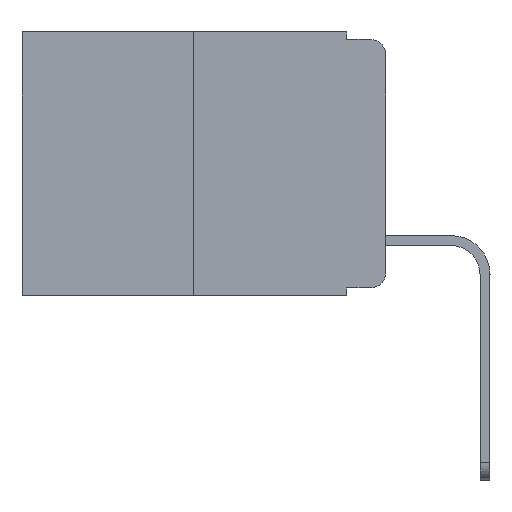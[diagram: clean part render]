
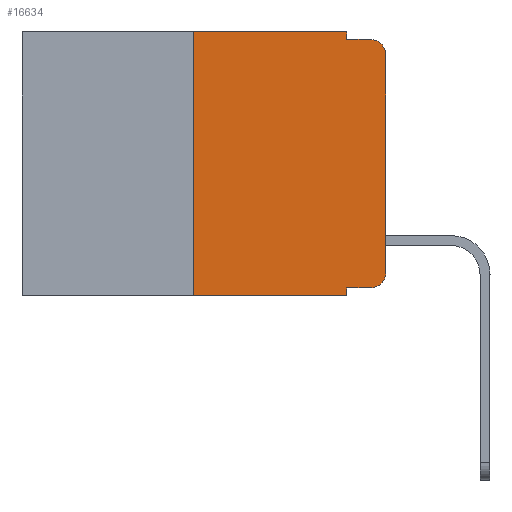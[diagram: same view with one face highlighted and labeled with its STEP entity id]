
A CAD part, left-side view. The second image highlights one B-rep face of the part: STEP entity #16634.
In plain terms, the highlighted planar face has unit normal (-1, 0, 0).
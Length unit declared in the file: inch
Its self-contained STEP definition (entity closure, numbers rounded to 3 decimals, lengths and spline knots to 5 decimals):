
#29 = VERTEX_POINT ( 'NONE', #22123 ) ;
#219 = LINE ( 'NONE', #21294, #9144 ) ;
#659 = ORIENTED_EDGE ( 'NONE', *, *, #23972, .F. ) ;
#1076 = CARTESIAN_POINT ( 'NONE',  ( 0., 0., 0. ) ) ;
#1132 = EDGE_CURVE ( 'NONE', #6059, #8301, #13253, .T. ) ;
#1584 = FACE_OUTER_BOUND ( 'NONE', #11433, .T. ) ;
#1598 = DIRECTION ( 'NONE',  ( -1., 0., 0. ) ) ;
#1832 = CARTESIAN_POINT ( 'NONE',  ( 0., 0.051, -0.01 ) ) ;
#2442 = VERTEX_POINT ( 'NONE', #19924 ) ;
#2556 = ORIENTED_EDGE ( 'NONE', *, *, #23384, .F. ) ;
#2822 = EDGE_CURVE ( 'NONE', #29, #23884, #219, .T. ) ;
#2874 = DIRECTION ( 'NONE',  ( 0., 0., -1. ) ) ;
#3214 = LINE ( 'NONE', #7345, #19552 ) ;
#3276 = DIRECTION ( 'NONE',  ( 0., -1., 0. ) ) ;
#4627 = CARTESIAN_POINT ( 'NONE',  ( 0., 0.051, -0.01 ) ) ;
#4629 = DIRECTION ( 'NONE',  ( 0., 0., -1. ) ) ;
#5206 = AXIS2_PLACEMENT_3D ( 'NONE', #10555, #16416, #2874 ) ;
#5526 = EDGE_CURVE ( 'NONE', #20418, #12722, #3214, .T. ) ;
#5607 = ORIENTED_EDGE ( 'NONE', *, *, #2822, .F. ) ;
#5917 = VECTOR ( 'NONE', #21841, 39.37008 ) ;
#6059 = VERTEX_POINT ( 'NONE', #24143 ) ;
#6416 = CARTESIAN_POINT ( 'NONE',  ( 0., 0.051, 0. ) ) ;
#6904 = VERTEX_POINT ( 'NONE', #23178 ) ;
#7303 = DIRECTION ( 'NONE',  ( 0., -1., 0. ) ) ;
#7345 = CARTESIAN_POINT ( 'NONE',  ( 0., 0.051, -0.333 ) ) ;
#7667 = DIRECTION ( 'NONE',  ( 1., 0., 0. ) ) ;
#7975 = CARTESIAN_POINT ( 'NONE',  ( 0., 0.25, 0. ) ) ;
#8301 = VERTEX_POINT ( 'NONE', #24394 ) ;
#9144 = VECTOR ( 'NONE', #9492, 39.37008 ) ;
#9200 = ORIENTED_EDGE ( 'NONE', *, *, #20712, .F. ) ;
#9492 = DIRECTION ( 'NONE',  ( 0., 0., 1. ) ) ;
#9667 = ORIENTED_EDGE ( 'NONE', *, *, #12054, .T. ) ;
#9822 = CARTESIAN_POINT ( 'NONE',  ( 0., 0.473, 0. ) ) ;
#9974 = AXIS2_PLACEMENT_3D ( 'NONE', #23070, #1598, #13242 ) ;
#10404 = CARTESIAN_POINT ( 'NONE',  ( 0., 0.051, 0. ) ) ;
#10523 = LINE ( 'NONE', #6416, #5917 ) ;
#10555 = CARTESIAN_POINT ( 'NONE',  ( 0., 0.02, -0.03 ) ) ;
#10673 = CIRCLE ( 'NONE', #9974, 0.02 ) ;
#11012 = VERTEX_POINT ( 'NONE', #4627 ) ;
#11121 = CARTESIAN_POINT ( 'NONE',  ( 0., 0.473, 0. ) ) ;
#11306 = DIRECTION ( 'NONE',  ( 0., -1., 0. ) ) ;
#11433 = EDGE_LOOP ( 'NONE', ( #9667, #17217, #9200, #2556, #20068, #5607, #19666, #659, #20910, #21505 ) ) ;
#11683 = VERTEX_POINT ( 'NONE', #16560 ) ;
#11777 = EDGE_CURVE ( 'NONE', #23884, #2442, #16621, .T. ) ;
#12054 = EDGE_CURVE ( 'NONE', #11683, #6059, #13211, .T. ) ;
#12722 = VERTEX_POINT ( 'NONE', #25110 ) ;
#13155 = CARTESIAN_POINT ( 'NONE',  ( 0., 0.473, -0.343 ) ) ;
#13211 = LINE ( 'NONE', #1076, #14444 ) ;
#13242 = DIRECTION ( 'NONE',  ( 0., 0., -1. ) ) ;
#13253 = CIRCLE ( 'NONE', #5206, 0.02 ) ;
#13723 = LINE ( 'NONE', #1832, #15301 ) ;
#14444 = VECTOR ( 'NONE', #18397, 39.37008 ) ;
#15301 = VECTOR ( 'NONE', #15362, 39.37008 ) ;
#15362 = DIRECTION ( 'NONE',  ( 0., -1., 0. ) ) ;
#15476 = VECTOR ( 'NONE', #4629, 39.37008 ) ;
#15696 = PLANE ( 'NONE',  #18304 ) ;
#16416 = DIRECTION ( 'NONE',  ( -1., 0., 0. ) ) ;
#16560 = CARTESIAN_POINT ( 'NONE',  ( 0., 0., -0.313 ) ) ;
#16621 = LINE ( 'NONE', #11121, #20907 ) ;
#16634 = ADVANCED_FACE ( 'NONE', ( #1584 ), #15696, .F. ) ;
#17202 = VECTOR ( 'NONE', #7303, 39.37008 ) ;
#17217 = ORIENTED_EDGE ( 'NONE', *, *, #1132, .T. ) ;
#18304 = AXIS2_PLACEMENT_3D ( 'NONE', #9822, #7667, #19456 ) ;
#18397 = DIRECTION ( 'NONE',  ( 0., 0., 1. ) ) ;
#18964 = EDGE_CURVE ( 'NONE', #12722, #11683, #10673, .T. ) ;
#19456 = DIRECTION ( 'NONE',  ( 0., 0., -1. ) ) ;
#19552 = VECTOR ( 'NONE', #11306, 39.37008 ) ;
#19666 = ORIENTED_EDGE ( 'NONE', *, *, #25426, .T. ) ;
#19924 = CARTESIAN_POINT ( 'NONE',  ( 0., 0.051, 0. ) ) ;
#20068 = ORIENTED_EDGE ( 'NONE', *, *, #11777, .F. ) ;
#20110 = LINE ( 'NONE', #10404, #15476 ) ;
#20418 = VERTEX_POINT ( 'NONE', #20440 ) ;
#20440 = CARTESIAN_POINT ( 'NONE',  ( 0., 0.051, -0.333 ) ) ;
#20712 = EDGE_CURVE ( 'NONE', #11012, #8301, #13723, .T. ) ;
#20907 = VECTOR ( 'NONE', #3276, 39.37008 ) ;
#20910 = ORIENTED_EDGE ( 'NONE', *, *, #5526, .T. ) ;
#21294 = CARTESIAN_POINT ( 'NONE',  ( 0., 0.25, 0. ) ) ;
#21505 = ORIENTED_EDGE ( 'NONE', *, *, #18964, .T. ) ;
#21841 = DIRECTION ( 'NONE',  ( 0., 0., -1. ) ) ;
#22123 = CARTESIAN_POINT ( 'NONE',  ( 0., 0.25, -0.343 ) ) ;
#23070 = CARTESIAN_POINT ( 'NONE',  ( 0., 0.02, -0.313 ) ) ;
#23178 = CARTESIAN_POINT ( 'NONE',  ( 0., 0.051, -0.343 ) ) ;
#23384 = EDGE_CURVE ( 'NONE', #2442, #11012, #20110, .T. ) ;
#23884 = VERTEX_POINT ( 'NONE', #7975 ) ;
#23972 = EDGE_CURVE ( 'NONE', #20418, #6904, #10523, .T. ) ;
#24017 = LINE ( 'NONE', #13155, #17202 ) ;
#24143 = CARTESIAN_POINT ( 'NONE',  ( 0., 0., -0.03 ) ) ;
#24394 = CARTESIAN_POINT ( 'NONE',  ( 0., 0.02, -0.01 ) ) ;
#25110 = CARTESIAN_POINT ( 'NONE',  ( 0., 0.02, -0.333 ) ) ;
#25426 = EDGE_CURVE ( 'NONE', #29, #6904, #24017, .T. ) ;
